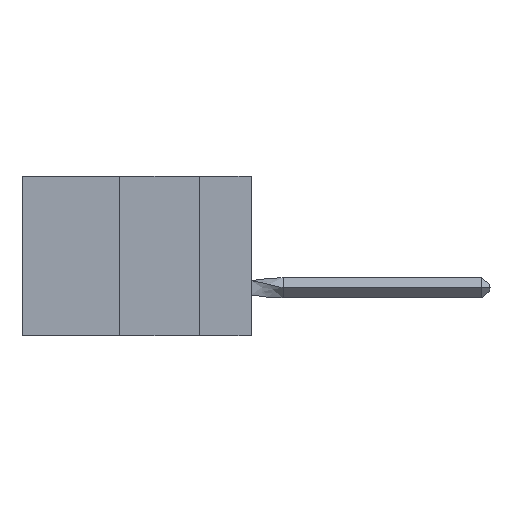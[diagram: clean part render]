
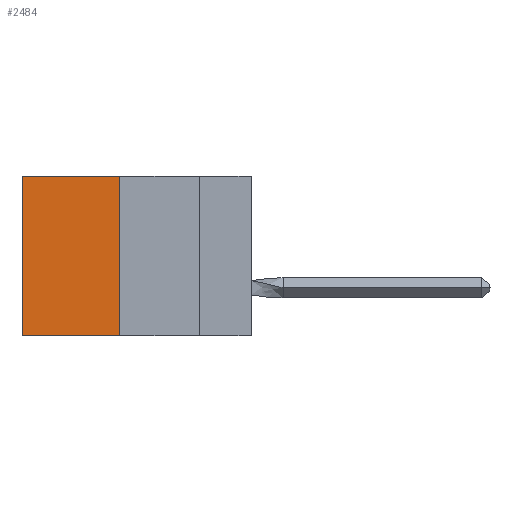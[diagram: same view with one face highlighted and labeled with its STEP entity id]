
A CAD part, left-side view. The second image highlights one B-rep face of the part: STEP entity #2484.
In plain terms, the highlighted planar face has unit normal (-1, 0, 0).
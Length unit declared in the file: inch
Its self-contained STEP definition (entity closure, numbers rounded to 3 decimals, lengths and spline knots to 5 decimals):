
#491 = VECTOR ( 'NONE', #25379, 39.37008 ) ;
#923 = CARTESIAN_POINT ( 'NONE',  ( 0.305, 0.413, -0.5 ) ) ;
#2484 = ADVANCED_FACE ( 'NONE', ( #15365 ), #3798, .F. ) ;
#3431 = CARTESIAN_POINT ( 'NONE',  ( 0.305, 0.413, -0.5 ) ) ;
#3798 = PLANE ( 'NONE',  #29648 ) ;
#5310 = VERTEX_POINT ( 'NONE', #26088 ) ;
#5549 = CARTESIAN_POINT ( 'NONE',  ( 0.305, 0.72, -0.5 ) ) ;
#6254 = DIRECTION ( 'NONE',  ( 0., 1., 0. ) ) ;
#7996 = ORIENTED_EDGE ( 'NONE', *, *, #35285, .T. ) ;
#8007 = EDGE_LOOP ( 'NONE', ( #31115, #24075, #10800, #7996 ) ) ;
#8358 = VERTEX_POINT ( 'NONE', #24777 ) ;
#9361 = LINE ( 'NONE', #16366, #22144 ) ;
#9914 = DIRECTION ( 'NONE',  ( 0., 1., 0. ) ) ;
#10792 = DIRECTION ( 'NONE',  ( 0., 0., -1. ) ) ;
#10800 = ORIENTED_EDGE ( 'NONE', *, *, #28475, .F. ) ;
#12892 = CARTESIAN_POINT ( 'NONE',  ( 0.305, 0.72, -0.5 ) ) ;
#15365 = FACE_OUTER_BOUND ( 'NONE', #8007, .T. ) ;
#15958 = CARTESIAN_POINT ( 'NONE',  ( 0.305, 0.413, 0. ) ) ;
#16366 = CARTESIAN_POINT ( 'NONE',  ( 0.305, 0.413, -0.5 ) ) ;
#18676 = LINE ( 'NONE', #923, #33694 ) ;
#19519 = CARTESIAN_POINT ( 'NONE',  ( 0.305, 0.413, 0. ) ) ;
#20206 = DIRECTION ( 'NONE',  ( 1., 0., 0. ) ) ;
#21408 = LINE ( 'NONE', #15958, #28057 ) ;
#22144 = VECTOR ( 'NONE', #10792, 39.37008 ) ;
#23450 = VERTEX_POINT ( 'NONE', #19519 ) ;
#24075 = ORIENTED_EDGE ( 'NONE', *, *, #26200, .F. ) ;
#24777 = CARTESIAN_POINT ( 'NONE',  ( 0.305, 0.72, 0. ) ) ;
#25379 = DIRECTION ( 'NONE',  ( 0., 0., -1. ) ) ;
#26088 = CARTESIAN_POINT ( 'NONE',  ( 0.305, 0.413, -0.5 ) ) ;
#26200 = EDGE_CURVE ( 'NONE', #5310, #33985, #18676, .T. ) ;
#28057 = VECTOR ( 'NONE', #9914, 39.37008 ) ;
#28475 = EDGE_CURVE ( 'NONE', #23450, #5310, #9361, .T. ) ;
#28979 = DIRECTION ( 'NONE',  ( 0., 0., -1. ) ) ;
#29027 = EDGE_CURVE ( 'NONE', #8358, #33985, #35429, .T. ) ;
#29648 = AXIS2_PLACEMENT_3D ( 'NONE', #3431, #20206, #28979 ) ;
#31115 = ORIENTED_EDGE ( 'NONE', *, *, #29027, .T. ) ;
#33694 = VECTOR ( 'NONE', #6254, 39.37008 ) ;
#33985 = VERTEX_POINT ( 'NONE', #12892 ) ;
#35285 = EDGE_CURVE ( 'NONE', #23450, #8358, #21408, .T. ) ;
#35429 = LINE ( 'NONE', #5549, #491 ) ;
